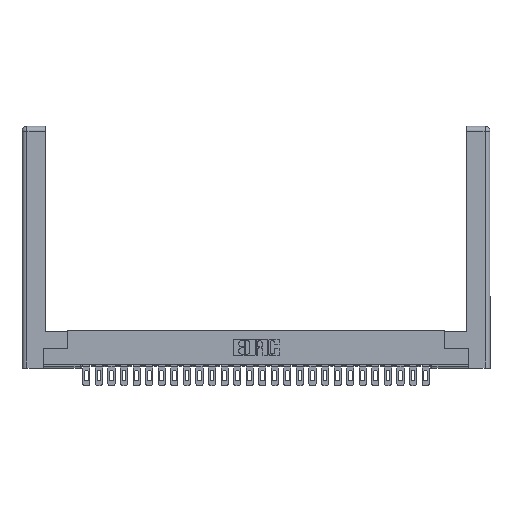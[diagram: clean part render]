
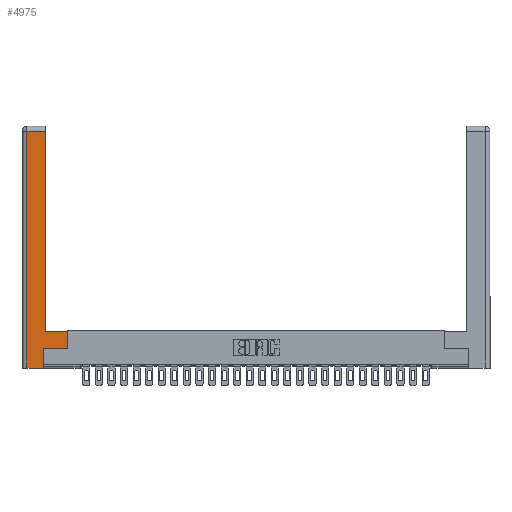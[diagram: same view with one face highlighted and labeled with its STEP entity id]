
A CAD part, top view. The second image highlights one B-rep face of the part: STEP entity #4975.
In plain terms, the highlighted planar face has unit normal (0, 0, 1).
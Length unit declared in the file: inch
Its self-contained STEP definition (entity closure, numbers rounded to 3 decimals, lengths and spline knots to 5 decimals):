
#152 = VERTEX_POINT ( 'NONE', #1027 ) ;
#1027 = CARTESIAN_POINT ( 'NONE',  ( 0.0615, 2.94, 0. ) ) ;
#1456 = EDGE_CURVE ( 'NONE', #22476, #15657, #23626, .T. ) ;
#2848 = DIRECTION ( 'NONE',  ( 0., 1., 0. ) ) ;
#3161 = CARTESIAN_POINT ( 'NONE',  ( 0.265, 0.245, 0. ) ) ;
#3288 = LINE ( 'NONE', #5048, #7102 ) ;
#3712 = VERTEX_POINT ( 'NONE', #3781 ) ;
#3713 = LINE ( 'NONE', #3858, #15070 ) ;
#3781 = CARTESIAN_POINT ( 'NONE',  ( 0.565, 0.245, 0. ) ) ;
#3858 = CARTESIAN_POINT ( 'NONE',  ( 0.265, 0., 0. ) ) ;
#4125 = EDGE_CURVE ( 'NONE', #5514, #25502, #3713, .T. ) ;
#4586 = ORIENTED_EDGE ( 'NONE', *, *, #4125, .T. ) ;
#4830 = VECTOR ( 'NONE', #20613, 39.37008 ) ;
#4975 = ADVANCED_FACE ( 'NONE', ( #8303 ), #17465, .F. ) ;
#5048 = CARTESIAN_POINT ( 'NONE',  ( 0.295, 3., 0. ) ) ;
#5135 = LINE ( 'NONE', #25486, #4830 ) ;
#5514 = VERTEX_POINT ( 'NONE', #15645 ) ;
#7102 = VECTOR ( 'NONE', #2848, 39.37008 ) ;
#7209 = VECTOR ( 'NONE', #23333, 39.37008 ) ;
#7573 = ORIENTED_EDGE ( 'NONE', *, *, #9503, .T. ) ;
#7923 = VERTEX_POINT ( 'NONE', #21165 ) ;
#8303 = FACE_OUTER_BOUND ( 'NONE', #17804, .T. ) ;
#8538 = AXIS2_PLACEMENT_3D ( 'NONE', #26466, #15254, #13606 ) ;
#9503 = EDGE_CURVE ( 'NONE', #15657, #7923, #3288, .T. ) ;
#10480 = EDGE_CURVE ( 'NONE', #7923, #152, #17480, .T. ) ;
#10809 = VECTOR ( 'NONE', #19719, 39.37008 ) ;
#11705 = LINE ( 'NONE', #27493, #15429 ) ;
#13585 = ORIENTED_EDGE ( 'NONE', *, *, #1456, .T. ) ;
#13606 = DIRECTION ( 'NONE',  ( -1., 0., 0. ) ) ;
#14018 = LINE ( 'NONE', #16366, #7209 ) ;
#14075 = DIRECTION ( 'NONE',  ( 0., 1., 0. ) ) ;
#14461 = CARTESIAN_POINT ( 'NONE',  ( 0.265, 0., 0. ) ) ;
#14464 = DIRECTION ( 'NONE',  ( 1., 0., 0. ) ) ;
#14665 = EDGE_CURVE ( 'NONE', #26892, #3712, #14018, .T. ) ;
#14681 = CARTESIAN_POINT ( 'NONE',  ( 0.565, 0.45, 0. ) ) ;
#15037 = EDGE_CURVE ( 'NONE', #152, #5514, #5135, .T. ) ;
#15070 = VECTOR ( 'NONE', #14464, 39.37008 ) ;
#15254 = DIRECTION ( 'NONE',  ( 0., 0., -1. ) ) ;
#15429 = VECTOR ( 'NONE', #14075, 39.37008 ) ;
#15645 = CARTESIAN_POINT ( 'NONE',  ( 0.0615, 0., 0. ) ) ;
#15657 = VERTEX_POINT ( 'NONE', #21316 ) ;
#16366 = CARTESIAN_POINT ( 'NONE',  ( 0.565, 0.245, 0. ) ) ;
#17058 = CARTESIAN_POINT ( 'NONE',  ( 0.565, 0.45, 0. ) ) ;
#17465 = PLANE ( 'NONE',  #8538 ) ;
#17480 = LINE ( 'NONE', #22070, #25092 ) ;
#17804 = EDGE_LOOP ( 'NONE', ( #7573, #18201, #28140, #4586, #18134, #18002, #18044, #13585 ) ) ;
#18002 = ORIENTED_EDGE ( 'NONE', *, *, #14665, .T. ) ;
#18044 = ORIENTED_EDGE ( 'NONE', *, *, #26640, .T. ) ;
#18134 = ORIENTED_EDGE ( 'NONE', *, *, #19184, .T. ) ;
#18201 = ORIENTED_EDGE ( 'NONE', *, *, #10480, .T. ) ;
#19184 = EDGE_CURVE ( 'NONE', #25502, #26892, #11705, .T. ) ;
#19424 = LINE ( 'NONE', #17058, #10809 ) ;
#19555 = DIRECTION ( 'NONE',  ( -1., 0., 0. ) ) ;
#19719 = DIRECTION ( 'NONE',  ( 0., 1., 0. ) ) ;
#20613 = DIRECTION ( 'NONE',  ( 0., -1., 0. ) ) ;
#21165 = CARTESIAN_POINT ( 'NONE',  ( 0.295, 2.94, 0. ) ) ;
#21247 = CARTESIAN_POINT ( 'NONE',  ( 0.295, 0.45, 0. ) ) ;
#21316 = CARTESIAN_POINT ( 'NONE',  ( 0.295, 0.45, 0. ) ) ;
#21407 = DIRECTION ( 'NONE',  ( -1., 0., 0. ) ) ;
#22070 = CARTESIAN_POINT ( 'NONE',  ( 0.0615, 2.94, 0. ) ) ;
#22476 = VERTEX_POINT ( 'NONE', #14681 ) ;
#23333 = DIRECTION ( 'NONE',  ( 1., 0., 0. ) ) ;
#23626 = LINE ( 'NONE', #21247, #28384 ) ;
#25092 = VECTOR ( 'NONE', #19555, 39.37008 ) ;
#25486 = CARTESIAN_POINT ( 'NONE',  ( 0.0615, 0., 0. ) ) ;
#25502 = VERTEX_POINT ( 'NONE', #14461 ) ;
#26466 = CARTESIAN_POINT ( 'NONE',  ( 0., 0., 0. ) ) ;
#26640 = EDGE_CURVE ( 'NONE', #3712, #22476, #19424, .T. ) ;
#26892 = VERTEX_POINT ( 'NONE', #3161 ) ;
#27493 = CARTESIAN_POINT ( 'NONE',  ( 0.265, 0.245, 0. ) ) ;
#28140 = ORIENTED_EDGE ( 'NONE', *, *, #15037, .T. ) ;
#28384 = VECTOR ( 'NONE', #21407, 39.37008 ) ;
